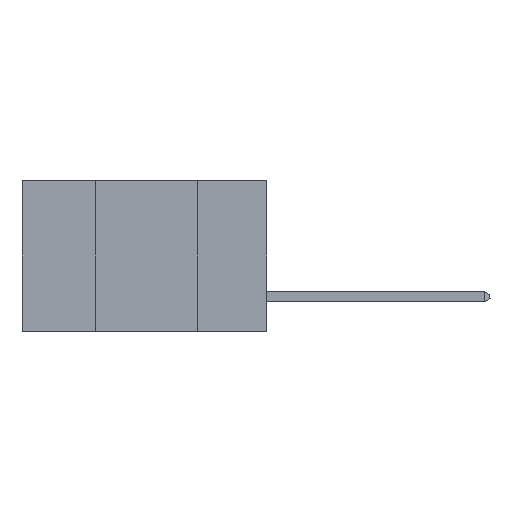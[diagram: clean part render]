
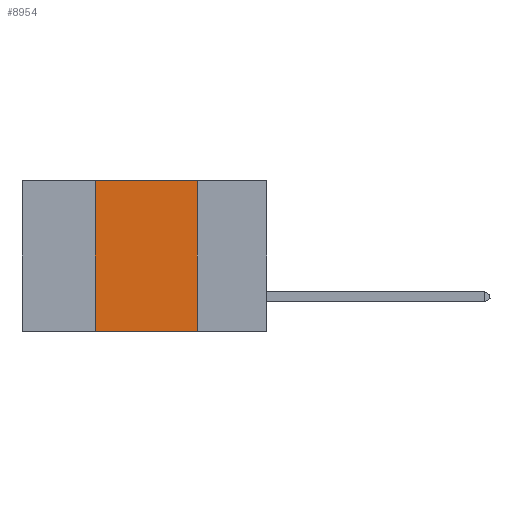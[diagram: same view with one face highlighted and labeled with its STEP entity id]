
A CAD part, left-side view. The second image highlights one B-rep face of the part: STEP entity #8954.
In plain terms, the highlighted planar face has unit normal (-1, 0, 0).
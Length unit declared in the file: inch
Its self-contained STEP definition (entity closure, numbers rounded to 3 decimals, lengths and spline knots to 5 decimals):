
#295 = VERTEX_POINT ( 'NONE', #20463 ) ;
#1353 = VERTEX_POINT ( 'NONE', #14512 ) ;
#1471 = VECTOR ( 'NONE', #22277, 39.37008 ) ;
#2419 = CARTESIAN_POINT ( 'NONE',  ( 0., 0.17, 0. ) ) ;
#2887 = EDGE_CURVE ( 'NONE', #1353, #17158, #6451, .T. ) ;
#3706 = DIRECTION ( 'NONE',  ( 0., 0., -1. ) ) ;
#3786 = AXIS2_PLACEMENT_3D ( 'NONE', #13588, #8273, #3706 ) ;
#4421 = EDGE_CURVE ( 'NONE', #1353, #295, #20713, .T. ) ;
#5886 = DIRECTION ( 'NONE',  ( 0., -1., 0. ) ) ;
#6451 = LINE ( 'NONE', #12175, #12373 ) ;
#6476 = CARTESIAN_POINT ( 'NONE',  ( 0., 0.6, 0. ) ) ;
#7187 = VECTOR ( 'NONE', #13189, 39.37008 ) ;
#7623 = LINE ( 'NONE', #2419, #13832 ) ;
#8273 = DIRECTION ( 'NONE',  ( 1., 0., 0. ) ) ;
#8954 = ADVANCED_FACE ( 'NONE', ( #19865 ), #12059, .F. ) ;
#10650 = EDGE_LOOP ( 'NONE', ( #19207, #18098, #12836, #12142 ) ) ;
#12059 = PLANE ( 'NONE',  #3786 ) ;
#12142 = ORIENTED_EDGE ( 'NONE', *, *, #2887, .T. ) ;
#12175 = CARTESIAN_POINT ( 'NONE',  ( 0., 0.6, -0.37 ) ) ;
#12373 = VECTOR ( 'NONE', #5886, 39.37008 ) ;
#12836 = ORIENTED_EDGE ( 'NONE', *, *, #4421, .F. ) ;
#13189 = DIRECTION ( 'NONE',  ( 0., -1., 0. ) ) ;
#13588 = CARTESIAN_POINT ( 'NONE',  ( 0., 0.6, 0. ) ) ;
#13832 = VECTOR ( 'NONE', #19714, 39.37008 ) ;
#14512 = CARTESIAN_POINT ( 'NONE',  ( 0., 0.42, -0.37 ) ) ;
#14676 = EDGE_CURVE ( 'NONE', #21644, #17158, #7623, .T. ) ;
#15480 = CARTESIAN_POINT ( 'NONE',  ( 0., 0.17, 0. ) ) ;
#17158 = VERTEX_POINT ( 'NONE', #22052 ) ;
#17214 = LINE ( 'NONE', #6476, #7187 ) ;
#18098 = ORIENTED_EDGE ( 'NONE', *, *, #19069, .F. ) ;
#19069 = EDGE_CURVE ( 'NONE', #295, #21644, #17214, .T. ) ;
#19207 = ORIENTED_EDGE ( 'NONE', *, *, #14676, .F. ) ;
#19714 = DIRECTION ( 'NONE',  ( 0., 0., -1. ) ) ;
#19865 = FACE_OUTER_BOUND ( 'NONE', #10650, .T. ) ;
#20463 = CARTESIAN_POINT ( 'NONE',  ( 0., 0.42, 0. ) ) ;
#20531 = CARTESIAN_POINT ( 'NONE',  ( 0., 0.42, 0. ) ) ;
#20713 = LINE ( 'NONE', #20531, #1471 ) ;
#21644 = VERTEX_POINT ( 'NONE', #15480 ) ;
#22052 = CARTESIAN_POINT ( 'NONE',  ( 0., 0.17, -0.37 ) ) ;
#22277 = DIRECTION ( 'NONE',  ( 0., 0., 1. ) ) ;
